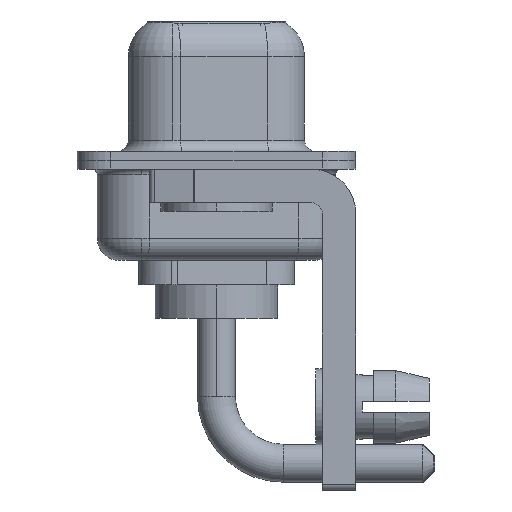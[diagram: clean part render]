
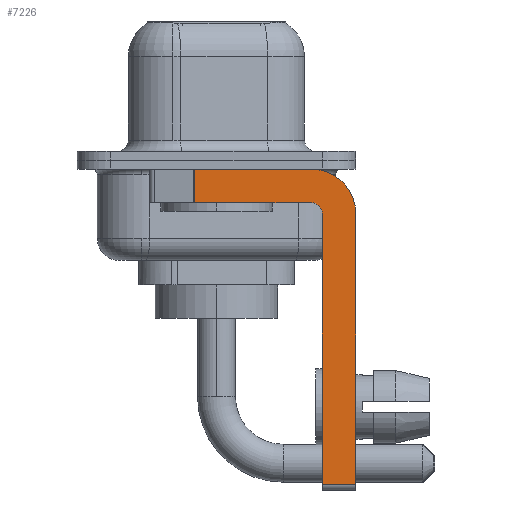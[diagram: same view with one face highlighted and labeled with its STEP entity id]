
A CAD part, left-side view. The second image highlights one B-rep face of the part: STEP entity #7226.
In plain terms, the highlighted planar face has unit normal (-1, 0, 0).
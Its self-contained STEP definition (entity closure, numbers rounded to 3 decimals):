
#233 = VECTOR ( 'NONE', #4076, 1000. ) ;
#399 = VECTOR ( 'NONE', #6908, 1000. ) ;
#400 = ORIENTED_EDGE ( 'NONE', *, *, #11422, .F. ) ;
#549 = FACE_OUTER_BOUND ( 'NONE', #9682, .T. ) ;
#1210 = DIRECTION ( 'NONE',  ( 0., 0., -1. ) ) ;
#1330 = VERTEX_POINT ( 'NONE', #13101 ) ;
#1665 = ORIENTED_EDGE ( 'NONE', *, *, #9909, .F. ) ;
#2236 = DIRECTION ( 'NONE',  ( 0., 0., 1. ) ) ;
#2455 = AXIS2_PLACEMENT_3D ( 'NONE', #6283, #7768, #12608 ) ;
#2483 = CARTESIAN_POINT ( 'NONE',  ( -2.9, -4.25, -2.4 ) ) ;
#2506 = CARTESIAN_POINT ( 'NONE',  ( -2.9, 0.978, -0.4 ) ) ;
#2682 = CIRCLE ( 'NONE', #7733, 0.5 ) ;
#2788 = VERTEX_POINT ( 'NONE', #14444 ) ;
#3139 = DIRECTION ( 'NONE',  ( 0., 1., 0. ) ) ;
#3296 = DIRECTION ( 'NONE',  ( 0., -1., 0. ) ) ;
#3403 = CARTESIAN_POINT ( 'NONE',  ( -2.9, -4.25, -1.9 ) ) ;
#3418 = LINE ( 'NONE', #3499, #399 ) ;
#3425 = CARTESIAN_POINT ( 'NONE',  ( -2.9, -4.25, -2.4 ) ) ;
#3486 = VECTOR ( 'NONE', #10512, 1000. ) ;
#3499 = CARTESIAN_POINT ( 'NONE',  ( -2.9, -4.75, -14.8 ) ) ;
#3604 = DIRECTION ( 'NONE',  ( 1., 0., 0. ) ) ;
#4076 = DIRECTION ( 'NONE',  ( 0., -1., 0. ) ) ;
#4245 = EDGE_CURVE ( 'NONE', #2788, #1330, #6975, .T. ) ;
#4263 = CARTESIAN_POINT ( 'NONE',  ( -2.9, 0.978, -1.9 ) ) ;
#4491 = CARTESIAN_POINT ( 'NONE',  ( -2.9, -4.25, -1.9 ) ) ;
#5034 = EDGE_CURVE ( 'NONE', #1330, #5347, #15372, .T. ) ;
#5347 = VERTEX_POINT ( 'NONE', #6626 ) ;
#5366 = DIRECTION ( 'NONE',  ( 0., 0., -1. ) ) ;
#5505 = EDGE_CURVE ( 'NONE', #10625, #2788, #7094, .T. ) ;
#6283 = CARTESIAN_POINT ( 'NONE',  ( -2.9, -4.25, -2.4 ) ) ;
#6327 = VERTEX_POINT ( 'NONE', #3403 ) ;
#6435 = ORIENTED_EDGE ( 'NONE', *, *, #13505, .T. ) ;
#6626 = CARTESIAN_POINT ( 'NONE',  ( -2.9, -6.25, -14.55 ) ) ;
#6877 = VERTEX_POINT ( 'NONE', #15505 ) ;
#6908 = DIRECTION ( 'NONE',  ( 0., 0., 1. ) ) ;
#6975 = CIRCLE ( 'NONE', #11003, 2. ) ;
#7079 = ORIENTED_EDGE ( 'NONE', *, *, #5034, .F. ) ;
#7094 = LINE ( 'NONE', #14243, #13451 ) ;
#7226 = ADVANCED_FACE ( 'NONE', ( #549 ), #15010, .F. ) ;
#7733 = AXIS2_PLACEMENT_3D ( 'NONE', #3425, #14366, #2236 ) ;
#7768 = DIRECTION ( 'NONE',  ( 1., 0., 0. ) ) ;
#8559 = ORIENTED_EDGE ( 'NONE', *, *, #14538, .T. ) ;
#8849 = LINE ( 'NONE', #14951, #233 ) ;
#8907 = EDGE_CURVE ( 'NONE', #6327, #10597, #14013, .T. ) ;
#9335 = VECTOR ( 'NONE', #5366, 1000. ) ;
#9570 = CARTESIAN_POINT ( 'NONE',  ( -2.9, 0.978, -1.9 ) ) ;
#9682 = EDGE_LOOP ( 'NONE', ( #11676, #6435, #13514, #400, #1665, #8559, #7079, #14055 ) ) ;
#9700 = VERTEX_POINT ( 'NONE', #11502 ) ;
#9909 = EDGE_CURVE ( 'NONE', #9700, #6877, #3418, .T. ) ;
#10512 = DIRECTION ( 'NONE',  ( 0., 0., -1. ) ) ;
#10597 = VERTEX_POINT ( 'NONE', #9570 ) ;
#10625 = VERTEX_POINT ( 'NONE', #2506 ) ;
#10877 = VECTOR ( 'NONE', #3139, 1000. ) ;
#11003 = AXIS2_PLACEMENT_3D ( 'NONE', #2483, #3604, #1210 ) ;
#11422 = EDGE_CURVE ( 'NONE', #6877, #6327, #2682, .T. ) ;
#11502 = CARTESIAN_POINT ( 'NONE',  ( -2.9, -4.75, -14.55 ) ) ;
#11676 = ORIENTED_EDGE ( 'NONE', *, *, #5505, .F. ) ;
#12608 = DIRECTION ( 'NONE',  ( 0., 0., -1. ) ) ;
#12735 = LINE ( 'NONE', #4263, #9335 ) ;
#13101 = CARTESIAN_POINT ( 'NONE',  ( -2.9, -6.25, -2.4 ) ) ;
#13451 = VECTOR ( 'NONE', #3296, 1000. ) ;
#13505 = EDGE_CURVE ( 'NONE', #10625, #10597, #12735, .T. ) ;
#13514 = ORIENTED_EDGE ( 'NONE', *, *, #8907, .F. ) ;
#14013 = LINE ( 'NONE', #4491, #10877 ) ;
#14055 = ORIENTED_EDGE ( 'NONE', *, *, #4245, .F. ) ;
#14243 = CARTESIAN_POINT ( 'NONE',  ( -2.9, 3., -0.4 ) ) ;
#14366 = DIRECTION ( 'NONE',  ( -1., 0., 0. ) ) ;
#14444 = CARTESIAN_POINT ( 'NONE',  ( -2.9, -4.25, -0.4 ) ) ;
#14538 = EDGE_CURVE ( 'NONE', #9700, #5347, #8849, .T. ) ;
#14951 = CARTESIAN_POINT ( 'NONE',  ( -2.9, -4.25, -14.55 ) ) ;
#15010 = PLANE ( 'NONE',  #2455 ) ;
#15372 = LINE ( 'NONE', #15608, #3486 ) ;
#15505 = CARTESIAN_POINT ( 'NONE',  ( -2.9, -4.75, -2.4 ) ) ;
#15608 = CARTESIAN_POINT ( 'NONE',  ( -2.9, -6.25, -2.4 ) ) ;
